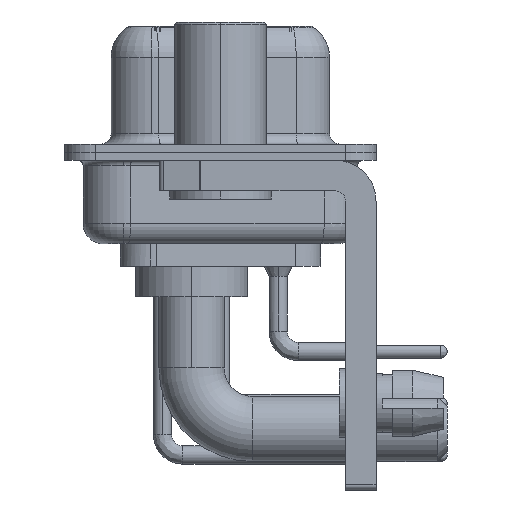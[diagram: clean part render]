
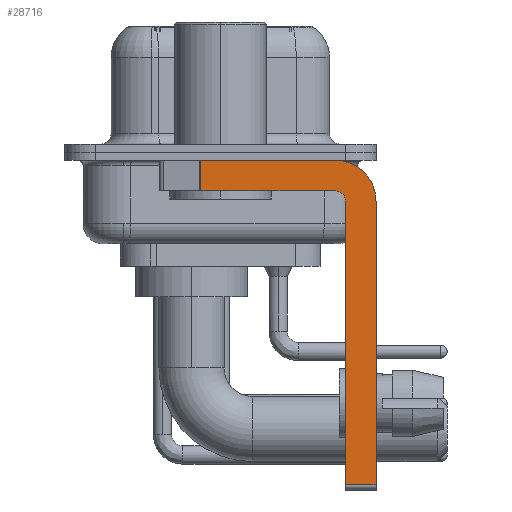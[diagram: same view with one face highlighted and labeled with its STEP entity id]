
A CAD part, left-side view. The second image highlights one B-rep face of the part: STEP entity #28716.
In plain terms, the highlighted planar face has unit normal (-1, 0, 0).
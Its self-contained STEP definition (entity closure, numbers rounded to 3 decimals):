
#133 = DIRECTION ( 'NONE',  ( 0., 0., -1. ) ) ;
#268 = EDGE_CURVE ( 'NONE', #9939, #12595, #15618, .T. ) ;
#995 = DIRECTION ( 'NONE',  ( 0., 0., -1. ) ) ;
#1085 = VECTOR ( 'NONE', #133, 1000. ) ;
#1469 = EDGE_CURVE ( 'NONE', #32717, #10806, #34442, .T. ) ;
#1583 = LINE ( 'NONE', #7332, #4117 ) ;
#2279 = VERTEX_POINT ( 'NONE', #16840 ) ;
#3395 = DIRECTION ( 'NONE',  ( -1., 0., 0. ) ) ;
#3601 = CARTESIAN_POINT ( 'NONE',  ( -2.9, -5.65, -1.9 ) ) ;
#3792 = DIRECTION ( 'NONE',  ( 1., 0., 0. ) ) ;
#3796 = LINE ( 'NONE', #26373, #9990 ) ;
#4117 = VECTOR ( 'NONE', #27147, 1000. ) ;
#5267 = CARTESIAN_POINT ( 'NONE',  ( -2.9, -6.15, -2.4 ) ) ;
#6066 = ORIENTED_EDGE ( 'NONE', *, *, #268, .F. ) ;
#6219 = AXIS2_PLACEMENT_3D ( 'NONE', #16590, #3395, #8094 ) ;
#6382 = DIRECTION ( 'NONE',  ( 0., -1., 0. ) ) ;
#6560 = PLANE ( 'NONE',  #18905 ) ;
#6853 = EDGE_CURVE ( 'NONE', #22624, #2279, #22181, .T. ) ;
#7126 = DIRECTION ( 'NONE',  ( 0., -1., 0. ) ) ;
#7332 = CARTESIAN_POINT ( 'NONE',  ( -2.9, 0.978, -1.9 ) ) ;
#7572 = AXIS2_PLACEMENT_3D ( 'NONE', #12168, #22877, #34231 ) ;
#8094 = DIRECTION ( 'NONE',  ( 0., 0., 1. ) ) ;
#9024 = CARTESIAN_POINT ( 'NONE',  ( -2.9, 0.978, -0.4 ) ) ;
#9711 = DIRECTION ( 'NONE',  ( 0., 1., 0. ) ) ;
#9939 = VERTEX_POINT ( 'NONE', #9024 ) ;
#9990 = VECTOR ( 'NONE', #6382, 1000. ) ;
#10483 = EDGE_CURVE ( 'NONE', #13841, #10806, #3796, .T. ) ;
#10806 = VERTEX_POINT ( 'NONE', #16874 ) ;
#12168 = CARTESIAN_POINT ( 'NONE',  ( -2.9, -5.65, -2.4 ) ) ;
#12323 = VECTOR ( 'NONE', #19377, 1000. ) ;
#12595 = VERTEX_POINT ( 'NONE', #14265 ) ;
#13841 = VERTEX_POINT ( 'NONE', #14272 ) ;
#14265 = CARTESIAN_POINT ( 'NONE',  ( -2.9, -5.65, -0.4 ) ) ;
#14272 = CARTESIAN_POINT ( 'NONE',  ( -2.9, -6.15, -16.35 ) ) ;
#15124 = ORIENTED_EDGE ( 'NONE', *, *, #10483, .T. ) ;
#15251 = CIRCLE ( 'NONE', #7572, 2. ) ;
#15425 = LINE ( 'NONE', #3601, #26983 ) ;
#15618 = LINE ( 'NONE', #18023, #22277 ) ;
#16027 = ORIENTED_EDGE ( 'NONE', *, *, #28296, .T. ) ;
#16590 = CARTESIAN_POINT ( 'NONE',  ( -2.9, -5.65, -2.4 ) ) ;
#16840 = CARTESIAN_POINT ( 'NONE',  ( -2.9, -5.65, -1.9 ) ) ;
#16874 = CARTESIAN_POINT ( 'NONE',  ( -2.9, -7.65, -16.35 ) ) ;
#17509 = EDGE_LOOP ( 'NONE', ( #6066, #16027, #33965, #34195, #20401, #15124, #22144, #20292 ) ) ;
#18023 = CARTESIAN_POINT ( 'NONE',  ( -2.9, 3., -0.4 ) ) ;
#18905 = AXIS2_PLACEMENT_3D ( 'NONE', #29164, #3792, #995 ) ;
#18943 = EDGE_CURVE ( 'NONE', #2279, #29884, #15425, .T. ) ;
#19377 = DIRECTION ( 'NONE',  ( 0., 0., 1. ) ) ;
#19401 = CARTESIAN_POINT ( 'NONE',  ( -2.9, -7.65, -2.4 ) ) ;
#20292 = ORIENTED_EDGE ( 'NONE', *, *, #26949, .F. ) ;
#20401 = ORIENTED_EDGE ( 'NONE', *, *, #25458, .F. ) ;
#22144 = ORIENTED_EDGE ( 'NONE', *, *, #1469, .F. ) ;
#22181 = CIRCLE ( 'NONE', #6219, 0.5 ) ;
#22277 = VECTOR ( 'NONE', #7126, 1000. ) ;
#22624 = VERTEX_POINT ( 'NONE', #5267 ) ;
#22877 = DIRECTION ( 'NONE',  ( 1., 0., 0. ) ) ;
#25458 = EDGE_CURVE ( 'NONE', #13841, #22624, #30164, .T. ) ;
#26373 = CARTESIAN_POINT ( 'NONE',  ( -2.9, -5.65, -16.35 ) ) ;
#26949 = EDGE_CURVE ( 'NONE', #12595, #32717, #15251, .T. ) ;
#26983 = VECTOR ( 'NONE', #9711, 1000. ) ;
#27147 = DIRECTION ( 'NONE',  ( 0., 0., -1. ) ) ;
#27188 = CARTESIAN_POINT ( 'NONE',  ( -2.9, -6.15, -16.6 ) ) ;
#28296 = EDGE_CURVE ( 'NONE', #9939, #29884, #1583, .T. ) ;
#28716 = ADVANCED_FACE ( 'NONE', ( #31592 ), #6560, .F. ) ;
#29164 = CARTESIAN_POINT ( 'NONE',  ( -2.9, -5.65, -2.4 ) ) ;
#29884 = VERTEX_POINT ( 'NONE', #34565 ) ;
#30164 = LINE ( 'NONE', #27188, #12323 ) ;
#31592 = FACE_OUTER_BOUND ( 'NONE', #17509, .T. ) ;
#32717 = VERTEX_POINT ( 'NONE', #36456 ) ;
#33965 = ORIENTED_EDGE ( 'NONE', *, *, #18943, .F. ) ;
#34195 = ORIENTED_EDGE ( 'NONE', *, *, #6853, .F. ) ;
#34231 = DIRECTION ( 'NONE',  ( 0., 0., -1. ) ) ;
#34442 = LINE ( 'NONE', #19401, #1085 ) ;
#34565 = CARTESIAN_POINT ( 'NONE',  ( -2.9, 0.978, -1.9 ) ) ;
#36456 = CARTESIAN_POINT ( 'NONE',  ( -2.9, -7.65, -2.4 ) ) ;
